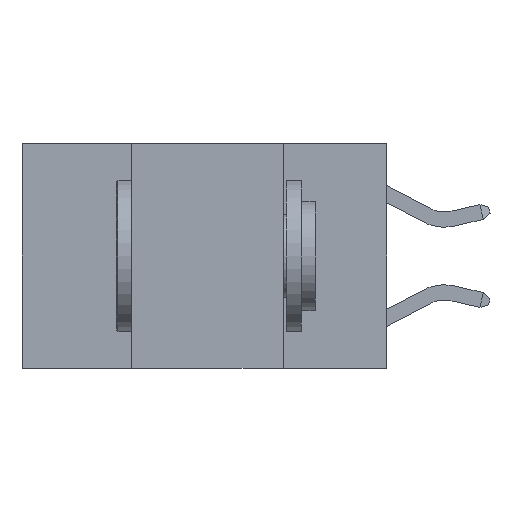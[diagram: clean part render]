
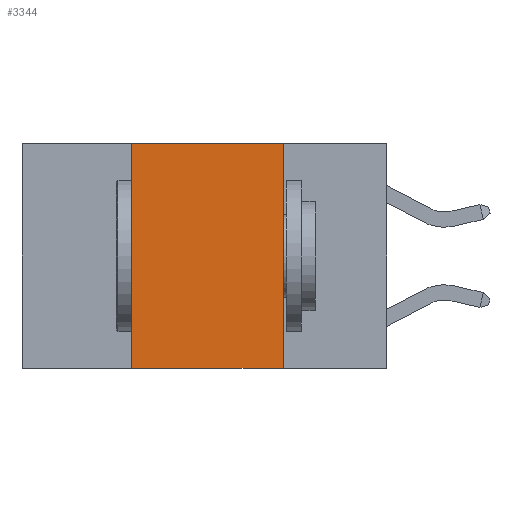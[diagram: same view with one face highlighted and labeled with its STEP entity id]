
A CAD part, left-side view. The second image highlights one B-rep face of the part: STEP entity #3344.
In plain terms, the highlighted planar face has unit normal (-1, 0, 0).
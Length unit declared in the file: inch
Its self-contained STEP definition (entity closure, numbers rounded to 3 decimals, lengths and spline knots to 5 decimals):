
#121 = LINE ( 'NONE', #17092, #3478 ) ;
#513 = DIRECTION ( 'NONE',  ( 0., 0., -1. ) ) ;
#533 = DIRECTION ( 'NONE',  ( 1., 0., 0. ) ) ;
#587 = PLANE ( 'NONE',  #15821 ) ;
#599 = ORIENTED_EDGE ( 'NONE', *, *, #15906, .T. ) ;
#607 = CARTESIAN_POINT ( 'NONE',  ( 0., 0.6, 0. ) ) ;
#864 = ORIENTED_EDGE ( 'NONE', *, *, #14062, .F. ) ;
#1014 = DIRECTION ( 'NONE',  ( 0., 0., -1. ) ) ;
#1126 = DIRECTION ( 'NONE',  ( 0., 0., 1. ) ) ;
#1176 = EDGE_LOOP ( 'NONE', ( #12708, #864, #18403, #599 ) ) ;
#2369 = CARTESIAN_POINT ( 'NONE',  ( 0., 0.6, 0. ) ) ;
#3344 = ADVANCED_FACE ( 'NONE', ( #15632 ), #587, .F. ) ;
#3478 = VECTOR ( 'NONE', #1126, 39.37008 ) ;
#3860 = CARTESIAN_POINT ( 'NONE',  ( 0., 0.17, 0. ) ) ;
#5536 = VERTEX_POINT ( 'NONE', #3860 ) ;
#8387 = DIRECTION ( 'NONE',  ( 0., -1., 0. ) ) ;
#10985 = CARTESIAN_POINT ( 'NONE',  ( 0., 0.17, -0.37 ) ) ;
#11265 = LINE ( 'NONE', #19452, #19218 ) ;
#12057 = LINE ( 'NONE', #2369, #19971 ) ;
#12708 = ORIENTED_EDGE ( 'NONE', *, *, #18013, .F. ) ;
#13536 = VERTEX_POINT ( 'NONE', #15273 ) ;
#14062 = EDGE_CURVE ( 'NONE', #13536, #5536, #12057, .T. ) ;
#14341 = VERTEX_POINT ( 'NONE', #10985 ) ;
#15095 = CARTESIAN_POINT ( 'NONE',  ( 0., 0.42, -0.37 ) ) ;
#15273 = CARTESIAN_POINT ( 'NONE',  ( 0., 0.42, 0. ) ) ;
#15314 = LINE ( 'NONE', #15401, #19013 ) ;
#15401 = CARTESIAN_POINT ( 'NONE',  ( 0., 0.17, 0. ) ) ;
#15632 = FACE_OUTER_BOUND ( 'NONE', #1176, .T. ) ;
#15821 = AXIS2_PLACEMENT_3D ( 'NONE', #607, #533, #513 ) ;
#15906 = EDGE_CURVE ( 'NONE', #20127, #14341, #11265, .T. ) ;
#16954 = EDGE_CURVE ( 'NONE', #20127, #13536, #121, .T. ) ;
#17092 = CARTESIAN_POINT ( 'NONE',  ( 0., 0.42, 0. ) ) ;
#18013 = EDGE_CURVE ( 'NONE', #5536, #14341, #15314, .T. ) ;
#18403 = ORIENTED_EDGE ( 'NONE', *, *, #16954, .F. ) ;
#19013 = VECTOR ( 'NONE', #1014, 39.37008 ) ;
#19218 = VECTOR ( 'NONE', #8387, 39.37008 ) ;
#19452 = CARTESIAN_POINT ( 'NONE',  ( 0., 0.6, -0.37 ) ) ;
#19901 = DIRECTION ( 'NONE',  ( 0., -1., 0. ) ) ;
#19971 = VECTOR ( 'NONE', #19901, 39.37008 ) ;
#20127 = VERTEX_POINT ( 'NONE', #15095 ) ;
